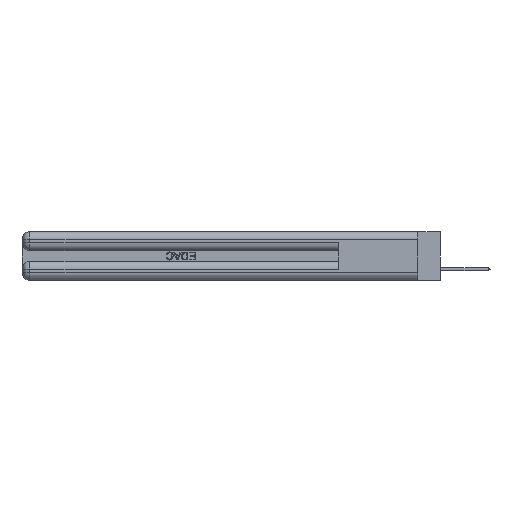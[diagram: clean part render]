
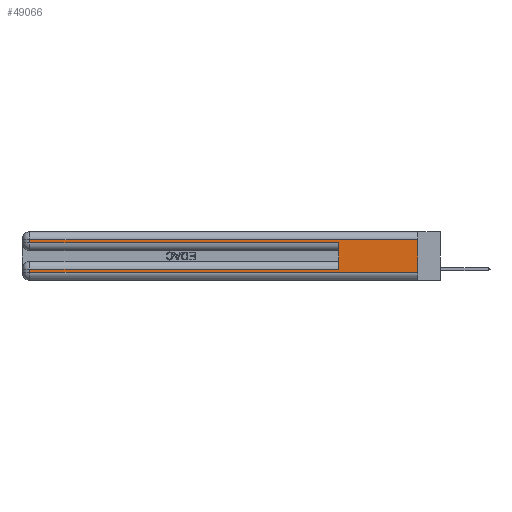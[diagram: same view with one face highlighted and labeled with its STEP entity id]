
A CAD part, left-side view. The second image highlights one B-rep face of the part: STEP entity #49066.
In plain terms, the highlighted planar face has unit normal (-1, 0, 0).
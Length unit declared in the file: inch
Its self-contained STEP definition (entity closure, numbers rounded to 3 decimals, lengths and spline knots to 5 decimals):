
#1152 = VECTOR ( 'NONE', #2741, 39.37008 ) ;
#1233 = VERTEX_POINT ( 'NONE', #35208 ) ;
#1664 = LINE ( 'NONE', #19732, #10671 ) ;
#2144 = CARTESIAN_POINT ( 'NONE',  ( 0., 0., 0.37 ) ) ;
#2741 = DIRECTION ( 'NONE',  ( 0., 0., -1. ) ) ;
#5009 = CARTESIAN_POINT ( 'NONE',  ( 0., 0., 0.06 ) ) ;
#5102 = VECTOR ( 'NONE', #7253, 39.37008 ) ;
#6885 = AXIS2_PLACEMENT_3D ( 'NONE', #2144, #10187, #28801 ) ;
#7253 = DIRECTION ( 'NONE',  ( 0., 0., 1. ) ) ;
#7459 = LINE ( 'NONE', #5009, #46756 ) ;
#8377 = CARTESIAN_POINT ( 'NONE',  ( 0., 2.94, 0.085 ) ) ;
#9007 = ORIENTED_EDGE ( 'NONE', *, *, #42234, .F. ) ;
#10187 = DIRECTION ( 'NONE',  ( 1., 0., 0. ) ) ;
#10671 = VECTOR ( 'NONE', #19896, 39.37008 ) ;
#11787 = DIRECTION ( 'NONE',  ( 0., 0., -1. ) ) ;
#12503 = ORIENTED_EDGE ( 'NONE', *, *, #39867, .T. ) ;
#13794 = EDGE_CURVE ( 'NONE', #26418, #44728, #7459, .T. ) ;
#14388 = CARTESIAN_POINT ( 'NONE',  ( 0., 0., 0.31 ) ) ;
#15219 = ORIENTED_EDGE ( 'NONE', *, *, #36825, .T. ) ;
#15228 = LINE ( 'NONE', #30063, #5102 ) ;
#15963 = VERTEX_POINT ( 'NONE', #27076 ) ;
#16761 = LINE ( 'NONE', #24225, #26896 ) ;
#16864 = VERTEX_POINT ( 'NONE', #21181 ) ;
#17258 = VECTOR ( 'NONE', #30962, 39.37008 ) ;
#19732 = CARTESIAN_POINT ( 'NONE',  ( 0., 2.94, 0.37 ) ) ;
#19896 = DIRECTION ( 'NONE',  ( 0., 0., -1. ) ) ;
#20275 = CARTESIAN_POINT ( 'NONE',  ( 0., 0., 0.285 ) ) ;
#21181 = CARTESIAN_POINT ( 'NONE',  ( 0., 2.94, 0.31 ) ) ;
#21442 = LINE ( 'NONE', #22207, #1152 ) ;
#22207 = CARTESIAN_POINT ( 'NONE',  ( 0., 0., 0.37 ) ) ;
#23736 = EDGE_CURVE ( 'NONE', #16864, #15963, #47272, .T. ) ;
#24225 = CARTESIAN_POINT ( 'NONE',  ( 0., 0., 0.085 ) ) ;
#24375 = ORIENTED_EDGE ( 'NONE', *, *, #23736, .T. ) ;
#24452 = EDGE_CURVE ( 'NONE', #15963, #41044, #38180, .T. ) ;
#24705 = CARTESIAN_POINT ( 'NONE',  ( 0., 0., 0.31 ) ) ;
#25520 = CARTESIAN_POINT ( 'NONE',  ( 0., 0.6, 0.285 ) ) ;
#25737 = DIRECTION ( 'NONE',  ( 0., 1., 0. ) ) ;
#26418 = VERTEX_POINT ( 'NONE', #41593 ) ;
#26896 = VECTOR ( 'NONE', #28378, 39.37008 ) ;
#27076 = CARTESIAN_POINT ( 'NONE',  ( 0., 2.94, 0.285 ) ) ;
#27560 = VECTOR ( 'NONE', #25737, 39.37008 ) ;
#28262 = VERTEX_POINT ( 'NONE', #8377 ) ;
#28378 = DIRECTION ( 'NONE',  ( 0., 1., 0. ) ) ;
#28801 = DIRECTION ( 'NONE',  ( 0., 0., -1. ) ) ;
#29683 = VERTEX_POINT ( 'NONE', #14388 ) ;
#30063 = CARTESIAN_POINT ( 'NONE',  ( 0., 0.6, 0.145 ) ) ;
#30962 = DIRECTION ( 'NONE',  ( 0., -1., 0. ) ) ;
#31072 = CARTESIAN_POINT ( 'NONE',  ( 0., 2.94, 0.37 ) ) ;
#31145 = VECTOR ( 'NONE', #11787, 39.37008 ) ;
#31627 = DIRECTION ( 'NONE',  ( 0., -1., 0. ) ) ;
#33771 = EDGE_LOOP ( 'NONE', ( #9007, #12503, #24375, #47613, #47830, #34439, #15219, #36452 ) ) ;
#34439 = ORIENTED_EDGE ( 'NONE', *, *, #43117, .T. ) ;
#35208 = CARTESIAN_POINT ( 'NONE',  ( 0., 0.6, 0.085 ) ) ;
#36452 = ORIENTED_EDGE ( 'NONE', *, *, #13794, .T. ) ;
#36825 = EDGE_CURVE ( 'NONE', #28262, #26418, #1664, .T. ) ;
#37825 = CARTESIAN_POINT ( 'NONE',  ( 0., 0., 0.06 ) ) ;
#38180 = LINE ( 'NONE', #20275, #17258 ) ;
#39867 = EDGE_CURVE ( 'NONE', #29683, #16864, #44302, .T. ) ;
#41044 = VERTEX_POINT ( 'NONE', #25520 ) ;
#41593 = CARTESIAN_POINT ( 'NONE',  ( 0., 2.94, 0.06 ) ) ;
#41881 = FACE_OUTER_BOUND ( 'NONE', #33771, .T. ) ;
#42234 = EDGE_CURVE ( 'NONE', #29683, #44728, #21442, .T. ) ;
#43117 = EDGE_CURVE ( 'NONE', #1233, #28262, #16761, .T. ) ;
#44302 = LINE ( 'NONE', #24705, #27560 ) ;
#44728 = VERTEX_POINT ( 'NONE', #37825 ) ;
#46756 = VECTOR ( 'NONE', #31627, 39.37008 ) ;
#47272 = LINE ( 'NONE', #31072, #31145 ) ;
#47561 = EDGE_CURVE ( 'NONE', #1233, #41044, #15228, .T. ) ;
#47613 = ORIENTED_EDGE ( 'NONE', *, *, #24452, .T. ) ;
#47820 = PLANE ( 'NONE',  #6885 ) ;
#47830 = ORIENTED_EDGE ( 'NONE', *, *, #47561, .F. ) ;
#49066 = ADVANCED_FACE ( 'NONE', ( #41881 ), #47820, .F. ) ;
